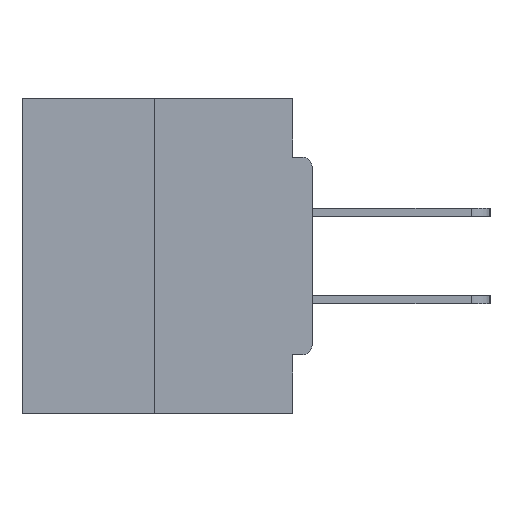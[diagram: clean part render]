
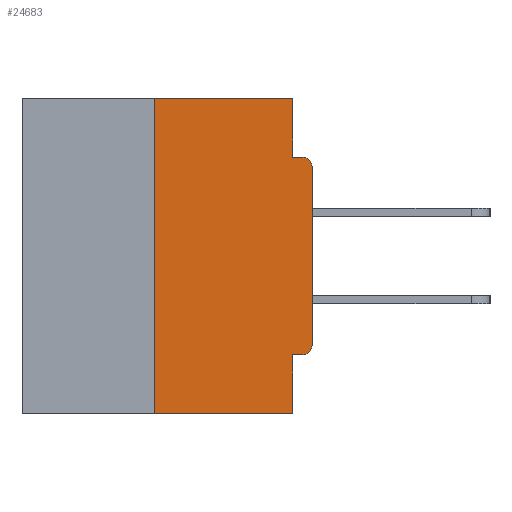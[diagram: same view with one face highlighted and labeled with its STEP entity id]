
A CAD part, left-side view. The second image highlights one B-rep face of the part: STEP entity #24683.
In plain terms, the highlighted planar face has unit normal (-1, 0, 0).
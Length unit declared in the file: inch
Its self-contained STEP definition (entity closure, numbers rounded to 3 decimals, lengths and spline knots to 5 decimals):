
#1548 = CARTESIAN_POINT ( 'NONE',  ( 0., 0., 0. ) ) ;
#1700 = CIRCLE ( 'NONE', #2547, 0.015 ) ;
#2205 = VECTOR ( 'NONE', #29200, 39.37008 ) ;
#2547 = AXIS2_PLACEMENT_3D ( 'NONE', #17673, #7839, #25329 ) ;
#2845 = CARTESIAN_POINT ( 'NONE',  ( 0., 0.25, 0. ) ) ;
#3700 = FACE_OUTER_BOUND ( 'NONE', #12208, .T. ) ;
#3714 = CARTESIAN_POINT ( 'NONE',  ( 0., 0.25, 0. ) ) ;
#3927 = LINE ( 'NONE', #15358, #10554 ) ;
#4055 = ORIENTED_EDGE ( 'NONE', *, *, #18139, .T. ) ;
#4148 = DIRECTION ( 'NONE',  ( 0., 0., 1. ) ) ;
#4414 = CARTESIAN_POINT ( 'NONE',  ( 0., 0.46, 0. ) ) ;
#4653 = LINE ( 'NONE', #28961, #10475 ) ;
#5665 = CIRCLE ( 'NONE', #11517, 0.015 ) ;
#5895 = ORIENTED_EDGE ( 'NONE', *, *, #28846, .F. ) ;
#6070 = VERTEX_POINT ( 'NONE', #17208 ) ;
#6532 = ORIENTED_EDGE ( 'NONE', *, *, #22184, .T. ) ;
#7839 = DIRECTION ( 'NONE',  ( -1., 0., 0. ) ) ;
#8314 = VERTEX_POINT ( 'NONE', #24699 ) ;
#8854 = LINE ( 'NONE', #3714, #10805 ) ;
#10407 = ORIENTED_EDGE ( 'NONE', *, *, #23026, .F. ) ;
#10475 = VECTOR ( 'NONE', #14087, 39.37008 ) ;
#10554 = VECTOR ( 'NONE', #17889, 39.37008 ) ;
#10805 = VECTOR ( 'NONE', #4148, 39.37008 ) ;
#11314 = VERTEX_POINT ( 'NONE', #20135 ) ;
#11517 = AXIS2_PLACEMENT_3D ( 'NONE', #12242, #16953, #12017 ) ;
#12017 = DIRECTION ( 'NONE',  ( 0., 0., -1. ) ) ;
#12208 = EDGE_LOOP ( 'NONE', ( #15227, #17534, #6532, #5895, #22087, #4055, #27198, #28285, #10407, #29416 ) ) ;
#12242 = CARTESIAN_POINT ( 'NONE',  ( 0., 0.015, -0.1085 ) ) ;
#13057 = DIRECTION ( 'NONE',  ( 1., 0., 0. ) ) ;
#13194 = VERTEX_POINT ( 'NONE', #2845 ) ;
#13395 = CARTESIAN_POINT ( 'NONE',  ( 0., 0.46, 0. ) ) ;
#13522 = VERTEX_POINT ( 'NONE', #25948 ) ;
#14087 = DIRECTION ( 'NONE',  ( 0., -1., 0. ) ) ;
#14476 = LINE ( 'NONE', #28263, #23504 ) ;
#15227 = ORIENTED_EDGE ( 'NONE', *, *, #25108, .F. ) ;
#15358 = CARTESIAN_POINT ( 'NONE',  ( 0., 0.031, 0. ) ) ;
#15388 = LINE ( 'NONE', #4414, #31442 ) ;
#15451 = AXIS2_PLACEMENT_3D ( 'NONE', #13395, #13057, #30550 ) ;
#15503 = CARTESIAN_POINT ( 'NONE',  ( 0., 0.015, -0.4065 ) ) ;
#15987 = DIRECTION ( 'NONE',  ( 0., -1., 0. ) ) ;
#16137 = VERTEX_POINT ( 'NONE', #24591 ) ;
#16837 = CARTESIAN_POINT ( 'NONE',  ( 0., 0.031, 0. ) ) ;
#16953 = DIRECTION ( 'NONE',  ( -1., 0., 0. ) ) ;
#17208 = CARTESIAN_POINT ( 'NONE',  ( 0., 0.031, -0.4065 ) ) ;
#17534 = ORIENTED_EDGE ( 'NONE', *, *, #32120, .F. ) ;
#17673 = CARTESIAN_POINT ( 'NONE',  ( 0., 0.015, -0.3915 ) ) ;
#17715 = EDGE_CURVE ( 'NONE', #30817, #16137, #5665, .T. ) ;
#17889 = DIRECTION ( 'NONE',  ( 0., 0., -1. ) ) ;
#18139 = EDGE_CURVE ( 'NONE', #23534, #29581, #1700, .T. ) ;
#19122 = VECTOR ( 'NONE', #29924, 39.37008 ) ;
#20135 = CARTESIAN_POINT ( 'NONE',  ( 0., 0.031, -0.5 ) ) ;
#20207 = LINE ( 'NONE', #26453, #2205 ) ;
#21824 = VERTEX_POINT ( 'NONE', #16837 ) ;
#22087 = ORIENTED_EDGE ( 'NONE', *, *, #26981, .F. ) ;
#22184 = EDGE_CURVE ( 'NONE', #8314, #11314, #14476, .T. ) ;
#22268 = LINE ( 'NONE', #27310, #19122 ) ;
#23026 = EDGE_CURVE ( 'NONE', #13522, #16137, #4653, .T. ) ;
#23504 = VECTOR ( 'NONE', #15987, 39.37008 ) ;
#23534 = VERTEX_POINT ( 'NONE', #15503 ) ;
#24591 = CARTESIAN_POINT ( 'NONE',  ( 0., 0.015, -0.0935 ) ) ;
#24683 = ADVANCED_FACE ( 'NONE', ( #3700 ), #28065, .F. ) ;
#24699 = CARTESIAN_POINT ( 'NONE',  ( 0., 0.25, -0.5 ) ) ;
#25108 = EDGE_CURVE ( 'NONE', #13194, #21824, #15388, .T. ) ;
#25329 = DIRECTION ( 'NONE',  ( 0., 0., -1. ) ) ;
#25948 = CARTESIAN_POINT ( 'NONE',  ( 0., 0.031, -0.0935 ) ) ;
#25993 = CARTESIAN_POINT ( 'NONE',  ( 0., 0., -0.3915 ) ) ;
#26453 = CARTESIAN_POINT ( 'NONE',  ( 0., 0.031, -0.5 ) ) ;
#26728 = EDGE_CURVE ( 'NONE', #21824, #13522, #3927, .T. ) ;
#26981 = EDGE_CURVE ( 'NONE', #23534, #6070, #22268, .T. ) ;
#27198 = ORIENTED_EDGE ( 'NONE', *, *, #30928, .T. ) ;
#27310 = CARTESIAN_POINT ( 'NONE',  ( 0., 0., -0.4065 ) ) ;
#28065 = PLANE ( 'NONE',  #15451 ) ;
#28263 = CARTESIAN_POINT ( 'NONE',  ( 0., 0.46, -0.5 ) ) ;
#28285 = ORIENTED_EDGE ( 'NONE', *, *, #17715, .T. ) ;
#28846 = EDGE_CURVE ( 'NONE', #6070, #11314, #20207, .T. ) ;
#28961 = CARTESIAN_POINT ( 'NONE',  ( 0., 0., -0.0935 ) ) ;
#29200 = DIRECTION ( 'NONE',  ( 0., 0., -1. ) ) ;
#29416 = ORIENTED_EDGE ( 'NONE', *, *, #26728, .F. ) ;
#29581 = VERTEX_POINT ( 'NONE', #25993 ) ;
#29869 = VECTOR ( 'NONE', #31849, 39.37008 ) ;
#29924 = DIRECTION ( 'NONE',  ( 0., 1., 0. ) ) ;
#30231 = LINE ( 'NONE', #1548, #29869 ) ;
#30511 = DIRECTION ( 'NONE',  ( 0., -1., 0. ) ) ;
#30550 = DIRECTION ( 'NONE',  ( 0., 0., -1. ) ) ;
#30817 = VERTEX_POINT ( 'NONE', #31084 ) ;
#30928 = EDGE_CURVE ( 'NONE', #29581, #30817, #30231, .T. ) ;
#31084 = CARTESIAN_POINT ( 'NONE',  ( 0., 0., -0.1085 ) ) ;
#31442 = VECTOR ( 'NONE', #30511, 39.37008 ) ;
#31849 = DIRECTION ( 'NONE',  ( 0., 0., 1. ) ) ;
#32120 = EDGE_CURVE ( 'NONE', #8314, #13194, #8854, .T. ) ;
